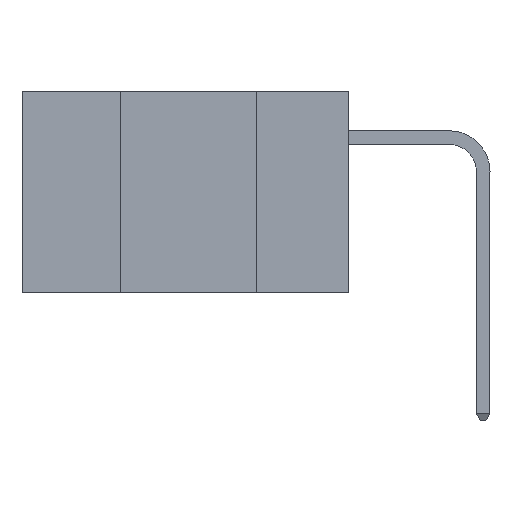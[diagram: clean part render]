
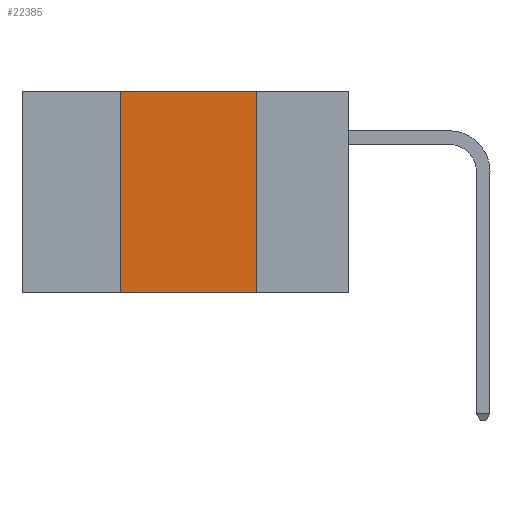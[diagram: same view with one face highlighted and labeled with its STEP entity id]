
A CAD part, left-side view. The second image highlights one B-rep face of the part: STEP entity #22385.
In plain terms, the highlighted planar face has unit normal (-1, 0, 0).
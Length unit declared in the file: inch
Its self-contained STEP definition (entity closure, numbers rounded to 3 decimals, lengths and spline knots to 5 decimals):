
#100 = CARTESIAN_POINT ( 'NONE',  ( 0., 0.17, 0. ) ) ;
#735 = EDGE_CURVE ( 'NONE', #11100, #6487, #11824, .T. ) ;
#1411 = EDGE_LOOP ( 'NONE', ( #4900, #21879, #15284, #19652 ) ) ;
#1487 = DIRECTION ( 'NONE',  ( 0., -1., 0. ) ) ;
#1863 = DIRECTION ( 'NONE',  ( 0., 0., -1. ) ) ;
#1959 = VECTOR ( 'NONE', #1863, 39.37008 ) ;
#1969 = VECTOR ( 'NONE', #20844, 39.37008 ) ;
#2082 = LINE ( 'NONE', #13427, #20894 ) ;
#4900 = ORIENTED_EDGE ( 'NONE', *, *, #735, .F. ) ;
#5268 = VECTOR ( 'NONE', #1487, 39.37008 ) ;
#5380 = PLANE ( 'NONE',  #13630 ) ;
#6487 = VERTEX_POINT ( 'NONE', #7791 ) ;
#6499 = FACE_OUTER_BOUND ( 'NONE', #1411, .T. ) ;
#7791 = CARTESIAN_POINT ( 'NONE',  ( 0., 0.17, -0.37 ) ) ;
#8774 = DIRECTION ( 'NONE',  ( 0., 0., -1. ) ) ;
#8906 = CARTESIAN_POINT ( 'NONE',  ( 0., 0.6, -0.37 ) ) ;
#10202 = LINE ( 'NONE', #8906, #1969 ) ;
#10734 = CARTESIAN_POINT ( 'NONE',  ( 0., 0.6, 0. ) ) ;
#11100 = VERTEX_POINT ( 'NONE', #14916 ) ;
#11824 = LINE ( 'NONE', #100, #1959 ) ;
#12389 = DIRECTION ( 'NONE',  ( 0., 0., 1. ) ) ;
#12425 = DIRECTION ( 'NONE',  ( 1., 0., 0. ) ) ;
#13427 = CARTESIAN_POINT ( 'NONE',  ( 0., 0.42, 0. ) ) ;
#13630 = AXIS2_PLACEMENT_3D ( 'NONE', #10734, #12425, #8774 ) ;
#14177 = CARTESIAN_POINT ( 'NONE',  ( 0., 0.42, 0. ) ) ;
#14916 = CARTESIAN_POINT ( 'NONE',  ( 0., 0.17, 0. ) ) ;
#15284 = ORIENTED_EDGE ( 'NONE', *, *, #16246, .F. ) ;
#15755 = VERTEX_POINT ( 'NONE', #14177 ) ;
#16246 = EDGE_CURVE ( 'NONE', #20745, #15755, #2082, .T. ) ;
#16726 = LINE ( 'NONE', #22406, #5268 ) ;
#17636 = CARTESIAN_POINT ( 'NONE',  ( 0., 0.42, -0.37 ) ) ;
#18728 = EDGE_CURVE ( 'NONE', #15755, #11100, #16726, .T. ) ;
#19438 = EDGE_CURVE ( 'NONE', #20745, #6487, #10202, .T. ) ;
#19652 = ORIENTED_EDGE ( 'NONE', *, *, #19438, .T. ) ;
#20745 = VERTEX_POINT ( 'NONE', #17636 ) ;
#20844 = DIRECTION ( 'NONE',  ( 0., -1., 0. ) ) ;
#20894 = VECTOR ( 'NONE', #12389, 39.37008 ) ;
#21879 = ORIENTED_EDGE ( 'NONE', *, *, #18728, .F. ) ;
#22385 = ADVANCED_FACE ( 'NONE', ( #6499 ), #5380, .F. ) ;
#22406 = CARTESIAN_POINT ( 'NONE',  ( 0., 0.6, 0. ) ) ;
